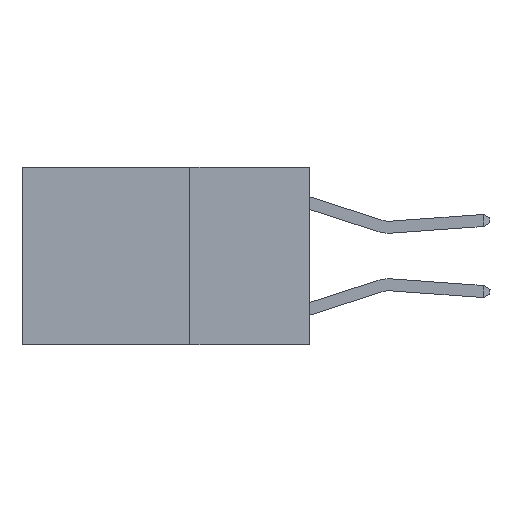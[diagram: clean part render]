
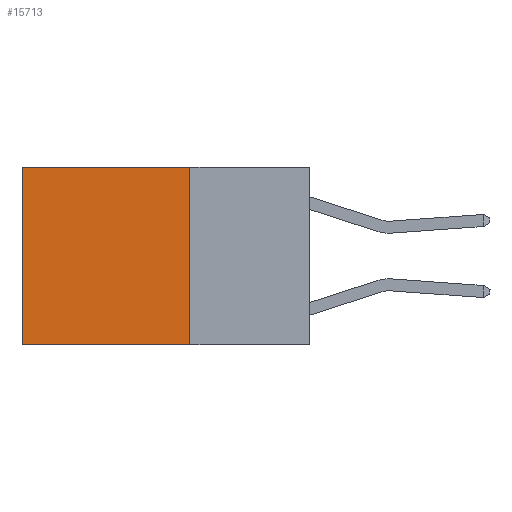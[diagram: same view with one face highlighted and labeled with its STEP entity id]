
A CAD part, left-side view. The second image highlights one B-rep face of the part: STEP entity #15713.
In plain terms, the highlighted planar face has unit normal (-1, 0, 0).
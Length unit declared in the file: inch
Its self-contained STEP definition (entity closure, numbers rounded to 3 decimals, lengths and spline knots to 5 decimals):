
#1507 = CARTESIAN_POINT ( 'NONE',  ( 0.2625, 0.25, -0.37 ) ) ;
#1520 = EDGE_CURVE ( 'NONE', #8589, #10424, #9580, .T. ) ;
#1708 = CARTESIAN_POINT ( 'NONE',  ( 0.2625, 0.25, 0. ) ) ;
#2889 = EDGE_LOOP ( 'NONE', ( #18566, #18013, #6254, #18383 ) ) ;
#3800 = DIRECTION ( 'NONE',  ( 0., 0., -1. ) ) ;
#4537 = EDGE_CURVE ( 'NONE', #10424, #17570, #24396, .T. ) ;
#4890 = CARTESIAN_POINT ( 'NONE',  ( 0.2625, 0.6, 0. ) ) ;
#5777 = CARTESIAN_POINT ( 'NONE',  ( 0.2625, 0.25, 0. ) ) ;
#6254 = ORIENTED_EDGE ( 'NONE', *, *, #1520, .F. ) ;
#7037 = DIRECTION ( 'NONE',  ( 0., 1., 0. ) ) ;
#7271 = CARTESIAN_POINT ( 'NONE',  ( 0.2625, 0.6, -0.37 ) ) ;
#7732 = EDGE_CURVE ( 'NONE', #26972, #17570, #22492, .T. ) ;
#8059 = FACE_OUTER_BOUND ( 'NONE', #2889, .T. ) ;
#8589 = VERTEX_POINT ( 'NONE', #5777 ) ;
#9332 = AXIS2_PLACEMENT_3D ( 'NONE', #9835, #24399, #11935 ) ;
#9580 = LINE ( 'NONE', #1708, #20030 ) ;
#9835 = CARTESIAN_POINT ( 'NONE',  ( 0.2625, 0.25, 0. ) ) ;
#10227 = VECTOR ( 'NONE', #7037, 39.37008 ) ;
#10424 = VERTEX_POINT ( 'NONE', #15418 ) ;
#10652 = CARTESIAN_POINT ( 'NONE',  ( 0.2625, 0.6, 0. ) ) ;
#11935 = DIRECTION ( 'NONE',  ( 0., 0., -1. ) ) ;
#13425 = CARTESIAN_POINT ( 'NONE',  ( 0.2625, 0.25, 0. ) ) ;
#15418 = CARTESIAN_POINT ( 'NONE',  ( 0.2625, 0.25, -0.37 ) ) ;
#15713 = ADVANCED_FACE ( 'NONE', ( #8059 ), #20220, .F. ) ;
#16970 = VECTOR ( 'NONE', #21668, 39.37008 ) ;
#17570 = VERTEX_POINT ( 'NONE', #7271 ) ;
#18013 = ORIENTED_EDGE ( 'NONE', *, *, #4537, .F. ) ;
#18126 = DIRECTION ( 'NONE',  ( 0., 1., 0. ) ) ;
#18383 = ORIENTED_EDGE ( 'NONE', *, *, #18870, .T. ) ;
#18566 = ORIENTED_EDGE ( 'NONE', *, *, #7732, .T. ) ;
#18870 = EDGE_CURVE ( 'NONE', #8589, #26972, #21291, .T. ) ;
#20030 = VECTOR ( 'NONE', #3800, 39.37008 ) ;
#20220 = PLANE ( 'NONE',  #9332 ) ;
#21291 = LINE ( 'NONE', #13425, #10227 ) ;
#21668 = DIRECTION ( 'NONE',  ( 0., 0., -1. ) ) ;
#22492 = LINE ( 'NONE', #4890, #16970 ) ;
#23736 = VECTOR ( 'NONE', #18126, 39.37008 ) ;
#24396 = LINE ( 'NONE', #1507, #23736 ) ;
#24399 = DIRECTION ( 'NONE',  ( 1., 0., 0. ) ) ;
#26972 = VERTEX_POINT ( 'NONE', #10652 ) ;
